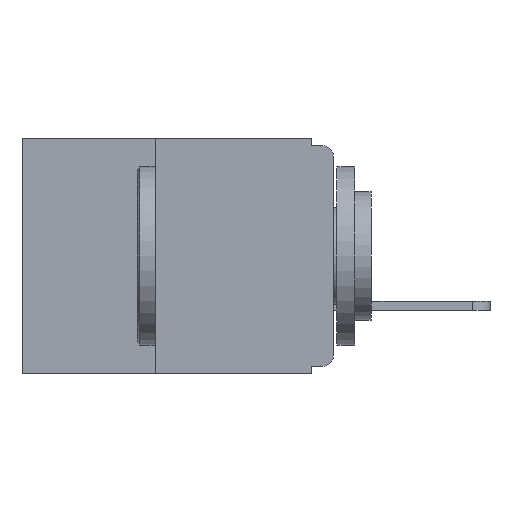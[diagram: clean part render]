
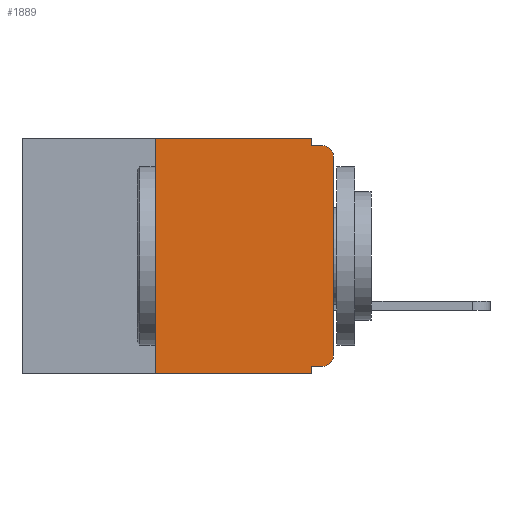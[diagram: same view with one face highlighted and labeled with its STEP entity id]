
A CAD part, left-side view. The second image highlights one B-rep face of the part: STEP entity #1889.
In plain terms, the highlighted planar face has unit normal (-1, 0, 0).
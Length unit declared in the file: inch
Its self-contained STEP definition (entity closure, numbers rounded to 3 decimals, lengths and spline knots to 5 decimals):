
#70 = VECTOR ( 'NONE', #5063, 39.37008 ) ;
#314 = ORIENTED_EDGE ( 'NONE', *, *, #3352, .F. ) ;
#763 = DIRECTION ( 'NONE',  ( 0., 0., -1. ) ) ;
#900 = LINE ( 'NONE', #5427, #11384 ) ;
#1376 = EDGE_CURVE ( 'NONE', #4169, #11019, #9250, .T. ) ;
#1889 = ADVANCED_FACE ( 'NONE', ( #8647 ), #7015, .F. ) ;
#1900 = ORIENTED_EDGE ( 'NONE', *, *, #7497, .F. ) ;
#1933 = CARTESIAN_POINT ( 'NONE',  ( 0., 0.25, 0. ) ) ;
#2213 = EDGE_CURVE ( 'NONE', #11019, #11496, #900, .T. ) ;
#2222 = VECTOR ( 'NONE', #5634, 39.37008 ) ;
#2251 = LINE ( 'NONE', #9620, #70 ) ;
#2755 = DIRECTION ( 'NONE',  ( -1., 0., 0. ) ) ;
#2808 = ORIENTED_EDGE ( 'NONE', *, *, #4667, .T. ) ;
#3096 = LINE ( 'NONE', #9398, #2222 ) ;
#3302 = CARTESIAN_POINT ( 'NONE',  ( 0., 0.437, -0.33 ) ) ;
#3352 = EDGE_CURVE ( 'NONE', #3363, #10600, #7059, .T. ) ;
#3363 = VERTEX_POINT ( 'NONE', #4367 ) ;
#3501 = DIRECTION ( 'NONE',  ( 0., 0., -1. ) ) ;
#3536 = EDGE_CURVE ( 'NONE', #11496, #3582, #5899, .T. ) ;
#3582 = VERTEX_POINT ( 'NONE', #3689 ) ;
#3644 = CARTESIAN_POINT ( 'NONE',  ( 0., 0.031, 0. ) ) ;
#3689 = CARTESIAN_POINT ( 'NONE',  ( 0., 0.015, -0.01 ) ) ;
#3787 = ORIENTED_EDGE ( 'NONE', *, *, #6649, .F. ) ;
#4124 = DIRECTION ( 'NONE',  ( 0., 0., -1. ) ) ;
#4143 = VECTOR ( 'NONE', #4124, 39.37008 ) ;
#4144 = DIRECTION ( 'NONE',  ( -1., 0., 0. ) ) ;
#4169 = VERTEX_POINT ( 'NONE', #7979 ) ;
#4367 = CARTESIAN_POINT ( 'NONE',  ( 0., 0.25, -0.33 ) ) ;
#4407 = DIRECTION ( 'NONE',  ( 0., 0., 1. ) ) ;
#4453 = CARTESIAN_POINT ( 'NONE',  ( 0., 0.25, -0.33 ) ) ;
#4627 = VECTOR ( 'NONE', #4407, 39.37008 ) ;
#4667 = EDGE_CURVE ( 'NONE', #3363, #6819, #11034, .T. ) ;
#5063 = DIRECTION ( 'NONE',  ( 0., -1., 0. ) ) ;
#5198 = CARTESIAN_POINT ( 'NONE',  ( 0., 0.031, -0.01 ) ) ;
#5368 = AXIS2_PLACEMENT_3D ( 'NONE', #6333, #2755, #10964 ) ;
#5427 = CARTESIAN_POINT ( 'NONE',  ( 0., 0., 0. ) ) ;
#5634 = DIRECTION ( 'NONE',  ( 0., -1., 0. ) ) ;
#5727 = ORIENTED_EDGE ( 'NONE', *, *, #3536, .T. ) ;
#5781 = EDGE_LOOP ( 'NONE', ( #9512, #5727, #10181, #3787, #1900, #314, #2808, #6670, #7905, #11250 ) ) ;
#5899 = CIRCLE ( 'NONE', #5368, 0.015 ) ;
#6023 = DIRECTION ( 'NONE',  ( 0., 1., 0. ) ) ;
#6101 = CARTESIAN_POINT ( 'NONE',  ( 0., 0., -0.32 ) ) ;
#6333 = CARTESIAN_POINT ( 'NONE',  ( 0., 0.015, -0.025 ) ) ;
#6363 = DIRECTION ( 'NONE',  ( 0., 0., 1. ) ) ;
#6649 = EDGE_CURVE ( 'NONE', #8773, #10364, #9544, .T. ) ;
#6670 = ORIENTED_EDGE ( 'NONE', *, *, #8819, .F. ) ;
#6819 = VERTEX_POINT ( 'NONE', #7464 ) ;
#6929 = CARTESIAN_POINT ( 'NONE',  ( 0., 0.015, -0.305 ) ) ;
#6967 = VERTEX_POINT ( 'NONE', #10472 ) ;
#7015 = PLANE ( 'NONE',  #11202 ) ;
#7059 = LINE ( 'NONE', #4453, #4627 ) ;
#7100 = EDGE_CURVE ( 'NONE', #4169, #6967, #10685, .T. ) ;
#7440 = VECTOR ( 'NONE', #8807, 39.37008 ) ;
#7464 = CARTESIAN_POINT ( 'NONE',  ( 0., 0.031, -0.33 ) ) ;
#7497 = EDGE_CURVE ( 'NONE', #10600, #8773, #3096, .T. ) ;
#7817 = CARTESIAN_POINT ( 'NONE',  ( 0., 0., -0.025 ) ) ;
#7839 = DIRECTION ( 'NONE',  ( 0., 0., -1. ) ) ;
#7905 = ORIENTED_EDGE ( 'NONE', *, *, #7100, .F. ) ;
#7979 = CARTESIAN_POINT ( 'NONE',  ( 0., 0.015, -0.32 ) ) ;
#8235 = VECTOR ( 'NONE', #6023, 39.37008 ) ;
#8647 = FACE_OUTER_BOUND ( 'NONE', #5781, .T. ) ;
#8773 = VERTEX_POINT ( 'NONE', #11553 ) ;
#8786 = EDGE_CURVE ( 'NONE', #10364, #3582, #2251, .T. ) ;
#8807 = DIRECTION ( 'NONE',  ( 0., -1., 0. ) ) ;
#8819 = EDGE_CURVE ( 'NONE', #6967, #6819, #9844, .T. ) ;
#8880 = DIRECTION ( 'NONE',  ( 1., 0., 0. ) ) ;
#8977 = CARTESIAN_POINT ( 'NONE',  ( 0., 0., -0.305 ) ) ;
#9250 = CIRCLE ( 'NONE', #9577, 0.015 ) ;
#9398 = CARTESIAN_POINT ( 'NONE',  ( 0., 0.437, 0. ) ) ;
#9512 = ORIENTED_EDGE ( 'NONE', *, *, #2213, .T. ) ;
#9544 = LINE ( 'NONE', #3644, #10996 ) ;
#9577 = AXIS2_PLACEMENT_3D ( 'NONE', #6929, #4144, #7839 ) ;
#9620 = CARTESIAN_POINT ( 'NONE',  ( 0., 0., -0.01 ) ) ;
#9840 = CARTESIAN_POINT ( 'NONE',  ( 0., 0.437, 0. ) ) ;
#9844 = LINE ( 'NONE', #10590, #4143 ) ;
#10181 = ORIENTED_EDGE ( 'NONE', *, *, #8786, .F. ) ;
#10364 = VERTEX_POINT ( 'NONE', #5198 ) ;
#10472 = CARTESIAN_POINT ( 'NONE',  ( 0., 0.031, -0.32 ) ) ;
#10590 = CARTESIAN_POINT ( 'NONE',  ( 0., 0.031, -0.33 ) ) ;
#10600 = VERTEX_POINT ( 'NONE', #1933 ) ;
#10685 = LINE ( 'NONE', #6101, #8235 ) ;
#10964 = DIRECTION ( 'NONE',  ( 0., 0., -1. ) ) ;
#10996 = VECTOR ( 'NONE', #763, 39.37008 ) ;
#11019 = VERTEX_POINT ( 'NONE', #8977 ) ;
#11034 = LINE ( 'NONE', #3302, #7440 ) ;
#11202 = AXIS2_PLACEMENT_3D ( 'NONE', #9840, #8880, #3501 ) ;
#11250 = ORIENTED_EDGE ( 'NONE', *, *, #1376, .T. ) ;
#11384 = VECTOR ( 'NONE', #6363, 39.37008 ) ;
#11496 = VERTEX_POINT ( 'NONE', #7817 ) ;
#11553 = CARTESIAN_POINT ( 'NONE',  ( 0., 0.031, 0. ) ) ;
